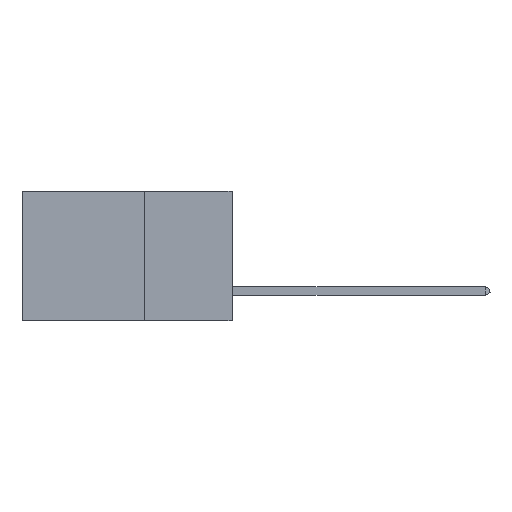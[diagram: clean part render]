
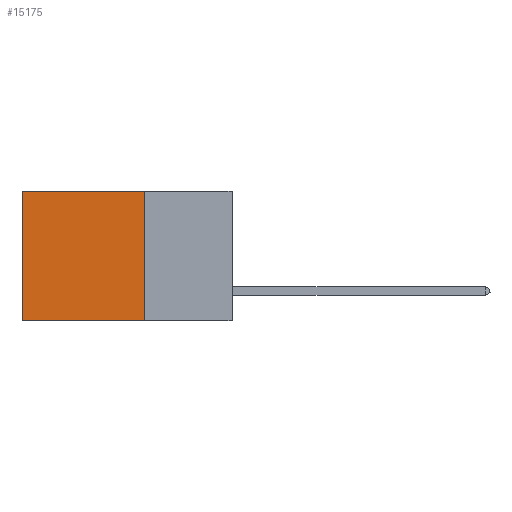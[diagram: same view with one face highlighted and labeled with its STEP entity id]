
A CAD part, left-side view. The second image highlights one B-rep face of the part: STEP entity #15175.
In plain terms, the highlighted planar face has unit normal (-1, 0, 0).
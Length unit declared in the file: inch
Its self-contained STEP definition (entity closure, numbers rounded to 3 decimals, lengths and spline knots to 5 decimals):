
#1453 = CARTESIAN_POINT ( 'NONE',  ( 0.2875, 0.25, -0.37 ) ) ;
#1664 = VERTEX_POINT ( 'NONE', #14574 ) ;
#2218 = VECTOR ( 'NONE', #6776, 39.37008 ) ;
#2288 = VECTOR ( 'NONE', #15708, 39.37008 ) ;
#2332 = VERTEX_POINT ( 'NONE', #1453 ) ;
#3203 = LINE ( 'NONE', #5579, #2288 ) ;
#3261 = FACE_OUTER_BOUND ( 'NONE', #12802, .T. ) ;
#4525 = VERTEX_POINT ( 'NONE', #17079 ) ;
#5001 = PLANE ( 'NONE',  #9643 ) ;
#5287 = EDGE_CURVE ( 'NONE', #2332, #15367, #15545, .T. ) ;
#5409 = VECTOR ( 'NONE', #8993, 39.37008 ) ;
#5579 = CARTESIAN_POINT ( 'NONE',  ( 0.2875, 0.6, 0. ) ) ;
#5839 = ORIENTED_EDGE ( 'NONE', *, *, #15656, .T. ) ;
#5941 = VECTOR ( 'NONE', #18512, 39.37008 ) ;
#6415 = DIRECTION ( 'NONE',  ( 0., 0., -1. ) ) ;
#6776 = DIRECTION ( 'NONE',  ( 0., 0., -1. ) ) ;
#7410 = ORIENTED_EDGE ( 'NONE', *, *, #16306, .T. ) ;
#8857 = LINE ( 'NONE', #16895, #5941 ) ;
#8993 = DIRECTION ( 'NONE',  ( 0., 1., 0. ) ) ;
#9643 = AXIS2_PLACEMENT_3D ( 'NONE', #14991, #15106, #6415 ) ;
#12802 = EDGE_LOOP ( 'NONE', ( #7410, #16211, #16464, #5839 ) ) ;
#13373 = CARTESIAN_POINT ( 'NONE',  ( 0.2875, 0.25, -0.37 ) ) ;
#14574 = CARTESIAN_POINT ( 'NONE',  ( 0.2875, 0.25, 0. ) ) ;
#14868 = LINE ( 'NONE', #16621, #2218 ) ;
#14991 = CARTESIAN_POINT ( 'NONE',  ( 0.2875, 0.25, 0. ) ) ;
#15106 = DIRECTION ( 'NONE',  ( 1., 0., 0. ) ) ;
#15175 = ADVANCED_FACE ( 'NONE', ( #3261 ), #5001, .F. ) ;
#15367 = VERTEX_POINT ( 'NONE', #17981 ) ;
#15545 = LINE ( 'NONE', #13373, #5409 ) ;
#15656 = EDGE_CURVE ( 'NONE', #1664, #4525, #8857, .T. ) ;
#15708 = DIRECTION ( 'NONE',  ( 0., 0., -1. ) ) ;
#16211 = ORIENTED_EDGE ( 'NONE', *, *, #5287, .F. ) ;
#16306 = EDGE_CURVE ( 'NONE', #4525, #15367, #3203, .T. ) ;
#16464 = ORIENTED_EDGE ( 'NONE', *, *, #17893, .F. ) ;
#16621 = CARTESIAN_POINT ( 'NONE',  ( 0.2875, 0.25, 0. ) ) ;
#16895 = CARTESIAN_POINT ( 'NONE',  ( 0.2875, 0.25, 0. ) ) ;
#17079 = CARTESIAN_POINT ( 'NONE',  ( 0.2875, 0.6, 0. ) ) ;
#17893 = EDGE_CURVE ( 'NONE', #1664, #2332, #14868, .T. ) ;
#17981 = CARTESIAN_POINT ( 'NONE',  ( 0.2875, 0.6, -0.37 ) ) ;
#18512 = DIRECTION ( 'NONE',  ( 0., 1., 0. ) ) ;
